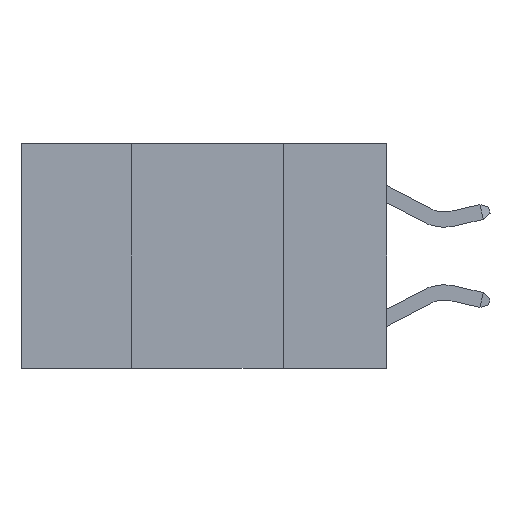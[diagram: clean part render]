
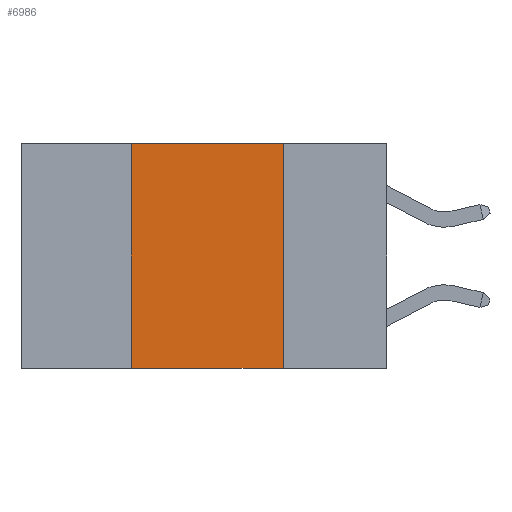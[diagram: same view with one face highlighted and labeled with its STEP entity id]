
A CAD part, left-side view. The second image highlights one B-rep face of the part: STEP entity #6986.
In plain terms, the highlighted planar face has unit normal (-1, 0, 0).
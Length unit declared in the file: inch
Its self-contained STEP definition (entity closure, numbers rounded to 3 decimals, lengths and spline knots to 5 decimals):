
#328 = DIRECTION ( 'NONE',  ( 0., 0., 1. ) ) ;
#1440 = LINE ( 'NONE', #3676, #13977 ) ;
#1698 = VERTEX_POINT ( 'NONE', #12626 ) ;
#2829 = EDGE_CURVE ( 'NONE', #8287, #8406, #19837, .T. ) ;
#2910 = LINE ( 'NONE', #19968, #19538 ) ;
#3059 = DIRECTION ( 'NONE',  ( 0., -1., 0. ) ) ;
#3676 = CARTESIAN_POINT ( 'NONE',  ( 0., 0.6, -0.37 ) ) ;
#3905 = ORIENTED_EDGE ( 'NONE', *, *, #2829, .F. ) ;
#4880 = CARTESIAN_POINT ( 'NONE',  ( 0., 0.42, 0. ) ) ;
#5073 = AXIS2_PLACEMENT_3D ( 'NONE', #19215, #20777, #11337 ) ;
#5309 = DIRECTION ( 'NONE',  ( 0., -1., 0. ) ) ;
#6986 = ADVANCED_FACE ( 'NONE', ( #8661 ), #9723, .F. ) ;
#7295 = DIRECTION ( 'NONE',  ( 0., 0., -1. ) ) ;
#8028 = EDGE_LOOP ( 'NONE', ( #19475, #16304, #3905, #13052 ) ) ;
#8287 = VERTEX_POINT ( 'NONE', #20445 ) ;
#8406 = VERTEX_POINT ( 'NONE', #4880 ) ;
#8661 = FACE_OUTER_BOUND ( 'NONE', #8028, .T. ) ;
#8789 = CARTESIAN_POINT ( 'NONE',  ( 0., 0.17, -0.37 ) ) ;
#9185 = VECTOR ( 'NONE', #328, 39.37008 ) ;
#9723 = PLANE ( 'NONE',  #5073 ) ;
#10345 = CARTESIAN_POINT ( 'NONE',  ( 0., 0.42, 0. ) ) ;
#11233 = EDGE_CURVE ( 'NONE', #8287, #19993, #1440, .T. ) ;
#11337 = DIRECTION ( 'NONE',  ( 0., 0., -1. ) ) ;
#12626 = CARTESIAN_POINT ( 'NONE',  ( 0., 0.17, 0. ) ) ;
#12675 = EDGE_CURVE ( 'NONE', #1698, #19993, #2910, .T. ) ;
#13052 = ORIENTED_EDGE ( 'NONE', *, *, #11233, .T. ) ;
#13977 = VECTOR ( 'NONE', #5309, 39.37008 ) ;
#15370 = VECTOR ( 'NONE', #3059, 39.37008 ) ;
#15953 = CARTESIAN_POINT ( 'NONE',  ( 0., 0.6, 0. ) ) ;
#16304 = ORIENTED_EDGE ( 'NONE', *, *, #19429, .F. ) ;
#19215 = CARTESIAN_POINT ( 'NONE',  ( 0., 0.6, 0. ) ) ;
#19429 = EDGE_CURVE ( 'NONE', #8406, #1698, #19564, .T. ) ;
#19475 = ORIENTED_EDGE ( 'NONE', *, *, #12675, .F. ) ;
#19538 = VECTOR ( 'NONE', #7295, 39.37008 ) ;
#19564 = LINE ( 'NONE', #15953, #15370 ) ;
#19837 = LINE ( 'NONE', #10345, #9185 ) ;
#19968 = CARTESIAN_POINT ( 'NONE',  ( 0., 0.17, 0. ) ) ;
#19993 = VERTEX_POINT ( 'NONE', #8789 ) ;
#20445 = CARTESIAN_POINT ( 'NONE',  ( 0., 0.42, -0.37 ) ) ;
#20777 = DIRECTION ( 'NONE',  ( 1., 0., 0. ) ) ;
